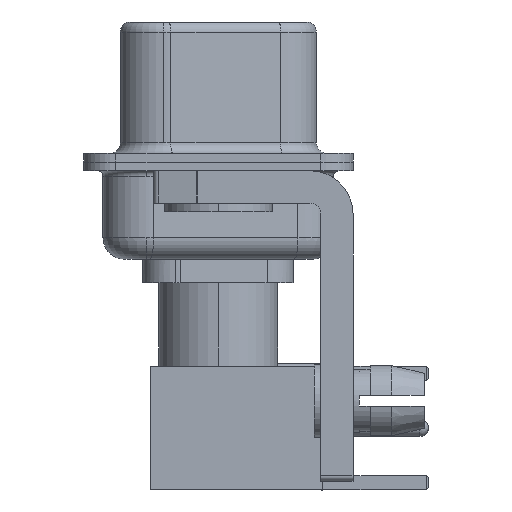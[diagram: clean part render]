
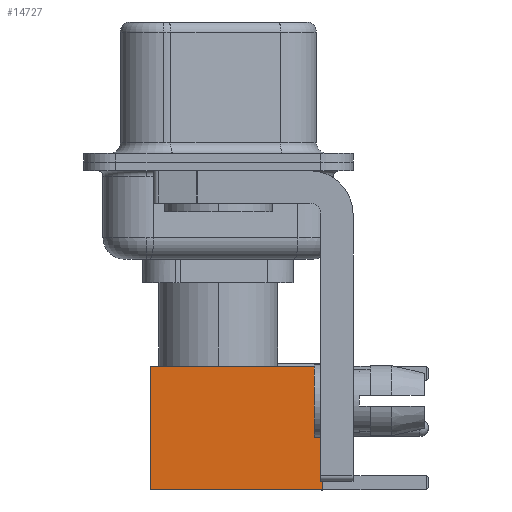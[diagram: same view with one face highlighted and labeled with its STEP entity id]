
A CAD part, left-side view. The second image highlights one B-rep face of the part: STEP entity #14727.
In plain terms, the highlighted face is planar.
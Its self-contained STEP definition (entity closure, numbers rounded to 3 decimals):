
#377 = DIRECTION ( 'NONE',  ( 0., 1., 0. ) ) ;
#1620 = DIRECTION ( 'NONE',  ( -1., 0., 0. ) ) ;
#2207 = CARTESIAN_POINT ( 'NONE',  ( 0., 2.875, 0. ) ) ;
#2368 = DIRECTION ( 'NONE',  ( -1., 0., 0. ) ) ;
#2675 = CARTESIAN_POINT ( 'NONE',  ( 2.875, 2.875, 0. ) ) ;
#3148 = VECTOR ( 'NONE', #6006, 1000. ) ;
#4249 = LINE ( 'NONE', #11567, #27541 ) ;
#5319 = FACE_OUTER_BOUND ( 'NONE', #7696, .T. ) ;
#5515 = CARTESIAN_POINT ( 'NONE',  ( -2.875, 2.875, 0. ) ) ;
#6006 = DIRECTION ( 'NONE',  ( 0., 0., -1. ) ) ;
#7475 = VERTEX_POINT ( 'NONE', #25664 ) ;
#7696 = EDGE_LOOP ( 'NONE', ( #24797, #11158, #16852, #16657 ) ) ;
#7944 = LINE ( 'NONE', #22055, #3148 ) ;
#7973 = DIRECTION ( 'NONE',  ( 0., 0., 1. ) ) ;
#8096 = VECTOR ( 'NONE', #2368, 1000. ) ;
#9669 = LINE ( 'NONE', #31358, #33204 ) ;
#10850 = VERTEX_POINT ( 'NONE', #11753 ) ;
#11158 = ORIENTED_EDGE ( 'NONE', *, *, #21350, .T. ) ;
#11567 = CARTESIAN_POINT ( 'NONE',  ( 0., 2.875, 8. ) ) ;
#11753 = CARTESIAN_POINT ( 'NONE',  ( 2.875, 2.875, 0. ) ) ;
#12468 = EDGE_CURVE ( 'NONE', #7475, #23583, #4249, .T. ) ;
#12660 = DIRECTION ( 'NONE',  ( 0., 0., -1. ) ) ;
#13492 = EDGE_CURVE ( 'NONE', #7475, #10850, #9669, .T. ) ;
#14727 = ADVANCED_FACE ( 'NONE', ( #5319 ), #16453, .T. ) ;
#16453 = PLANE ( 'NONE',  #25631 ) ;
#16657 = ORIENTED_EDGE ( 'NONE', *, *, #12468, .F. ) ;
#16852 = ORIENTED_EDGE ( 'NONE', *, *, #33512, .F. ) ;
#21350 = EDGE_CURVE ( 'NONE', #10850, #31692, #26553, .T. ) ;
#22055 = CARTESIAN_POINT ( 'NONE',  ( -2.875, 2.875, 0. ) ) ;
#23583 = VERTEX_POINT ( 'NONE', #33371 ) ;
#24797 = ORIENTED_EDGE ( 'NONE', *, *, #13492, .T. ) ;
#25631 = AXIS2_PLACEMENT_3D ( 'NONE', #2675, #377, #7973 ) ;
#25664 = CARTESIAN_POINT ( 'NONE',  ( 2.875, 2.875, 8. ) ) ;
#26553 = LINE ( 'NONE', #2207, #8096 ) ;
#27541 = VECTOR ( 'NONE', #1620, 1000. ) ;
#31358 = CARTESIAN_POINT ( 'NONE',  ( 2.875, 2.875, 0. ) ) ;
#31692 = VERTEX_POINT ( 'NONE', #5515 ) ;
#33204 = VECTOR ( 'NONE', #12660, 1000. ) ;
#33371 = CARTESIAN_POINT ( 'NONE',  ( -2.875, 2.875, 8. ) ) ;
#33512 = EDGE_CURVE ( 'NONE', #23583, #31692, #7944, .T. ) ;
